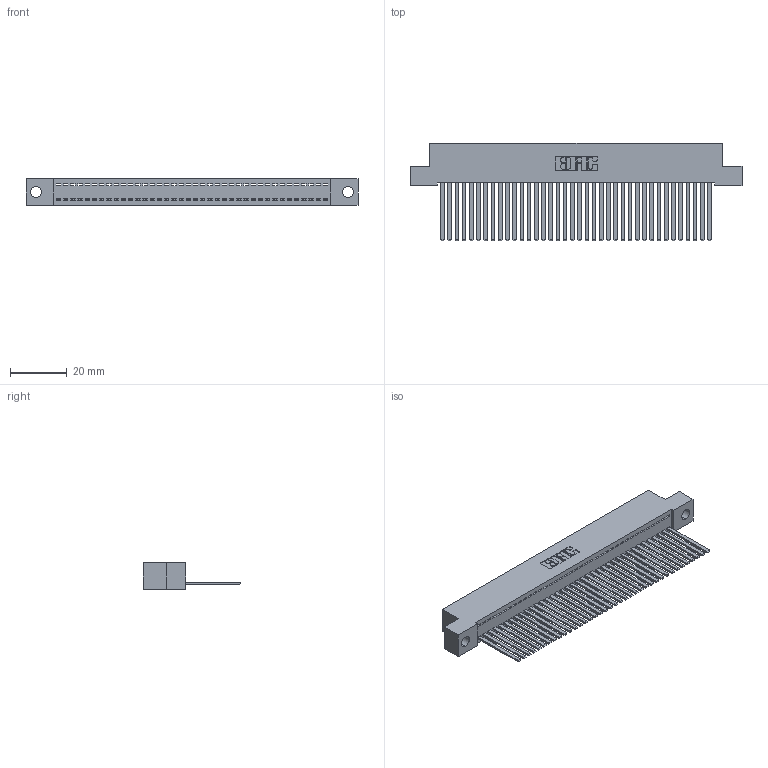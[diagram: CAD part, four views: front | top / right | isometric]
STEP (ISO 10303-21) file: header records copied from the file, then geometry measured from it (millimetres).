
FILE_DESCRIPTION (( 'STEP AP203' ), '1' );
FILE_NAME ('392-038-544-104.STEP', '2019-10-07T19:02:46', ( '' ), ( '' ), 'SwSTEP 2.0', 'SolidWorks 2016', '' );
FILE_SCHEMA (( 'CONFIG_CONTROL_DESIGN' ));
Length unit declared in the file: inch
Products named in the file (3): 392-038-544-104; 342 Part_.156 TH; 345-292-001_345-293-144
Assembly tree (39 placements, depth 2):
  392-038-544-104
    342 Part_.156 TH
    345-292-001_345-293-144  x38
Bounding box: 116.84 x 34.3 x 9.4 mm (x, y, z)
Volume: 10582.9 mm3; surface area: 16537.1 mm2
Topology: 39 solids, 39 shells, 2086 faces, 6303 edges, 4150 vertices
Faces by surface type: plane 1510, cylinder 576
Entity records: 23435 total; most frequent: CARTESIAN_POINT 4048, ORIENTED_EDGE 4022, DIRECTION 3419, EDGE_CURVE 2011, VECTOR 1887, LINE 1887, VERTEX_POINT 1338, AXIS2_PLACEMENT_3D 766
